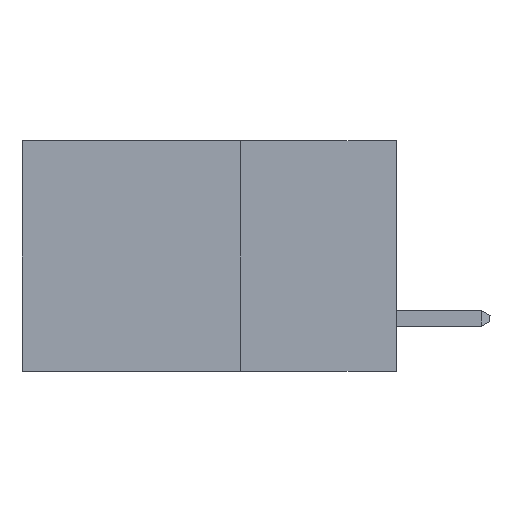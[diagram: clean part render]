
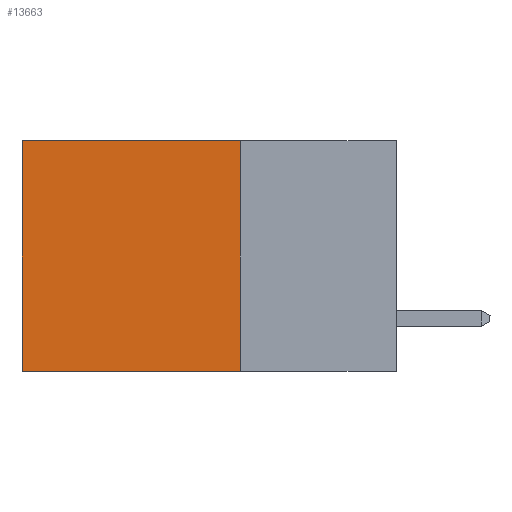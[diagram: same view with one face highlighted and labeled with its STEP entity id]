
A CAD part, left-side view. The second image highlights one B-rep face of the part: STEP entity #13663.
In plain terms, the highlighted planar face has unit normal (-1, 0, 0).
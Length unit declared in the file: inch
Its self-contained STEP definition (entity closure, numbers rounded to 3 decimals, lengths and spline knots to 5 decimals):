
#42 = DIRECTION ( 'NONE',  ( 0., 0., -1. ) ) ;
#2098 = VECTOR ( 'NONE', #12039, 39.37008 ) ;
#2787 = CARTESIAN_POINT ( 'NONE',  ( 0.2615, 0.25, -0.37 ) ) ;
#4046 = CARTESIAN_POINT ( 'NONE',  ( 0.2615, 0.25, -0.37 ) ) ;
#4324 = CARTESIAN_POINT ( 'NONE',  ( 0.2615, 0.25, -0.37 ) ) ;
#4430 = AXIS2_PLACEMENT_3D ( 'NONE', #4324, #8663, #42 ) ;
#4740 = CARTESIAN_POINT ( 'NONE',  ( 0.2615, 0.25, -0.37 ) ) ;
#5023 = LINE ( 'NONE', #13923, #2098 ) ;
#5378 = DIRECTION ( 'NONE',  ( 0., 0., -1. ) ) ;
#5860 = ORIENTED_EDGE ( 'NONE', *, *, #9652, .F. ) ;
#6249 = EDGE_CURVE ( 'NONE', #16549, #13123, #15719, .T. ) ;
#7671 = EDGE_LOOP ( 'NONE', ( #9378, #5860, #9698, #16157 ) ) ;
#7879 = VERTEX_POINT ( 'NONE', #17068 ) ;
#7989 = CARTESIAN_POINT ( 'NONE',  ( 0.2615, 0.6, 0. ) ) ;
#8156 = DIRECTION ( 'NONE',  ( 0., 0., -1. ) ) ;
#8663 = DIRECTION ( 'NONE',  ( 1., 0., 0. ) ) ;
#9106 = VECTOR ( 'NONE', #8156, 39.37008 ) ;
#9378 = ORIENTED_EDGE ( 'NONE', *, *, #6249, .T. ) ;
#9652 = EDGE_CURVE ( 'NONE', #10192, #13123, #14420, .T. ) ;
#9698 = ORIENTED_EDGE ( 'NONE', *, *, #17459, .F. ) ;
#10192 = VERTEX_POINT ( 'NONE', #4740 ) ;
#12039 = DIRECTION ( 'NONE',  ( 0., 1., 0. ) ) ;
#12392 = CARTESIAN_POINT ( 'NONE',  ( 0.2615, 0.6, -0.37 ) ) ;
#13009 = DIRECTION ( 'NONE',  ( 0., 1., 0. ) ) ;
#13038 = PLANE ( 'NONE',  #4430 ) ;
#13123 = VERTEX_POINT ( 'NONE', #12392 ) ;
#13663 = ADVANCED_FACE ( 'NONE', ( #17264 ), #13038, .F. ) ;
#13923 = CARTESIAN_POINT ( 'NONE',  ( 0.2615, 0.25, 0. ) ) ;
#14420 = LINE ( 'NONE', #2787, #15838 ) ;
#15719 = LINE ( 'NONE', #18545, #9106 ) ;
#15838 = VECTOR ( 'NONE', #13009, 39.37008 ) ;
#15997 = VECTOR ( 'NONE', #5378, 39.37008 ) ;
#16157 = ORIENTED_EDGE ( 'NONE', *, *, #16899, .T. ) ;
#16549 = VERTEX_POINT ( 'NONE', #7989 ) ;
#16899 = EDGE_CURVE ( 'NONE', #7879, #16549, #5023, .T. ) ;
#17068 = CARTESIAN_POINT ( 'NONE',  ( 0.2615, 0.25, 0. ) ) ;
#17264 = FACE_OUTER_BOUND ( 'NONE', #7671, .T. ) ;
#17459 = EDGE_CURVE ( 'NONE', #7879, #10192, #18219, .T. ) ;
#18219 = LINE ( 'NONE', #4046, #15997 ) ;
#18545 = CARTESIAN_POINT ( 'NONE',  ( 0.2615, 0.6, -0.37 ) ) ;
